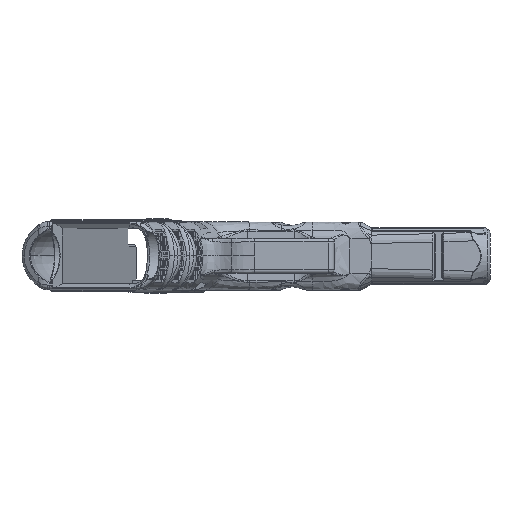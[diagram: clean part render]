
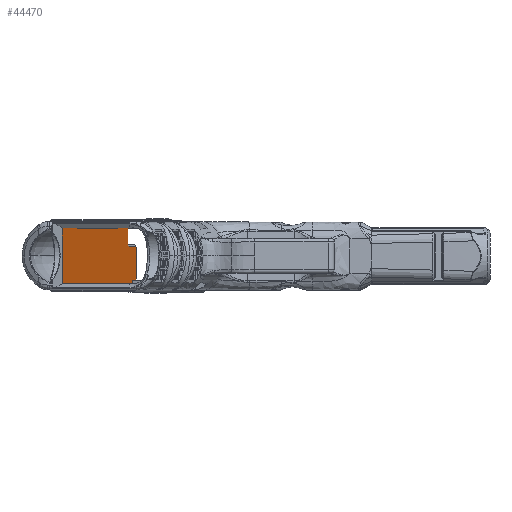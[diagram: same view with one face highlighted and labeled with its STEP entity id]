
A CAD part, top view. The second image highlights one B-rep face of the part: STEP entity #44470.
In plain terms, the highlighted planar face has unit normal (0.951, 0, 0.309).
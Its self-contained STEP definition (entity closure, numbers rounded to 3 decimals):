
#2195=LINE('',#99948,#4883);
#2961=LINE('',#152782,#5649);
#3145=LINE('',#160101,#5833);
#3148=LINE('',#160106,#5836);
#3153=LINE('',#160131,#5841);
#3154=LINE('',#160134,#5842);
#3155=LINE('',#160136,#5843);
#3156=LINE('',#160140,#5844);
#3157=LINE('',#160142,#5845);
#3158=LINE('',#160143,#5846);
#4883=VECTOR('',#52501,10.);
#5649=VECTOR('',#55797,10.);
#5833=VECTOR('',#56309,10.);
#5836=VECTOR('',#56316,10.);
#5841=VECTOR('',#56331,1000.);
#5842=VECTOR('',#56334,10.);
#5843=VECTOR('',#56335,10.);
#5844=VECTOR('',#56338,10.);
#5845=VECTOR('',#56339,10.);
#5846=VECTOR('',#56340,1000.);
#7071=PLANE('',#47829);
#8424=ELLIPSE('',#47830,0.536,0.51);
#10354=FACE_OUTER_BOUND('',#12789,.T.);
#12789=EDGE_LOOP('',(#39009,#39010,#39011,#39012,#39013,#39014,#39015,#39016,
#39017,#39018,#39019));
#18536=VERTEX_POINT('',#99830);
#18546=VERTEX_POINT('',#99929);
#19970=VERTEX_POINT('',#152779);
#19971=VERTEX_POINT('',#152781);
#20238=VERTEX_POINT('',#160095);
#20240=VERTEX_POINT('',#160099);
#20248=VERTEX_POINT('',#160133);
#20249=VERTEX_POINT('',#160135);
#20250=VERTEX_POINT('',#160137);
#20251=VERTEX_POINT('',#160139);
#20252=VERTEX_POINT('',#160141);
#24022=EDGE_CURVE('',#18536,#18546,#2195,.T.);
#26262=EDGE_CURVE('',#19970,#19971,#2961,.T.);
#26684=EDGE_CURVE('',#20238,#20240,#3145,.T.);
#26687=EDGE_CURVE('',#20240,#19971,#3148,.T.);
#26697=EDGE_CURVE('',#20238,#18536,#3153,.T.);
#26698=EDGE_CURVE('',#20248,#19970,#3154,.T.);
#26699=EDGE_CURVE('',#20249,#20248,#3155,.T.);
#26700=EDGE_CURVE('',#20250,#20249,#8424,.T.);
#26701=EDGE_CURVE('',#20251,#20250,#3156,.T.);
#26702=EDGE_CURVE('',#20252,#20251,#3157,.T.);
#26703=EDGE_CURVE('',#18546,#20252,#3158,.T.);
#39009=ORIENTED_EDGE('',*,*,#26697,.F.);
#39010=ORIENTED_EDGE('',*,*,#26684,.T.);
#39011=ORIENTED_EDGE('',*,*,#26687,.T.);
#39012=ORIENTED_EDGE('',*,*,#26262,.F.);
#39013=ORIENTED_EDGE('',*,*,#26698,.F.);
#39014=ORIENTED_EDGE('',*,*,#26699,.F.);
#39015=ORIENTED_EDGE('',*,*,#26700,.F.);
#39016=ORIENTED_EDGE('',*,*,#26701,.F.);
#39017=ORIENTED_EDGE('',*,*,#26702,.F.);
#39018=ORIENTED_EDGE('',*,*,#26703,.F.);
#39019=ORIENTED_EDGE('',*,*,#24022,.F.);
#44470=ADVANCED_FACE('',(#10354),#7071,.F.);
#47829=AXIS2_PLACEMENT_3D('',#160132,#56332,#56333);
#47830=AXIS2_PLACEMENT_3D('',#160138,#56336,#56337);
#52501=DIRECTION('',(0.,1.,0.));
#55797=DIRECTION('',(0.,-1.,0.));
#56309=DIRECTION('',(0.,1.,0.));
#56316=DIRECTION('',(0.309,0.,-0.951));
#56331=DIRECTION('',(-0.309,0.,0.951));
#56332=DIRECTION('center_axis',(-0.951,0.,
-0.309));
#56333=DIRECTION('ref_axis',(0.,1.,0.));
#56334=DIRECTION('',(-0.309,0.,0.951));
#56335=DIRECTION('',(0.,-1.,0.));
#56336=DIRECTION('center_axis',(-0.951,0.,
-0.309));
#56337=DIRECTION('ref_axis',(0.309,0.,-0.951));
#56338=DIRECTION('',(0.309,0.,-0.951));
#56339=DIRECTION('',(0.,-1.,0.));
#56340=DIRECTION('',(0.309,0.,-0.951));
#99830=CARTESIAN_POINT('',(2.236,-11.75,98.));
#99929=CARTESIAN_POINT('',(2.236,11.75,98.));
#99948=CARTESIAN_POINT('',(2.236,-18.375,98.));
#152779=CARTESIAN_POINT('',(33.331,-9.542,2.3));
#152781=CARTESIAN_POINT('',(33.331,-10.25,2.3));
#152782=CARTESIAN_POINT('',(33.331,-5.876,2.3));
#160095=CARTESIAN_POINT('',(31.8,-11.75,7.012));
#160099=CARTESIAN_POINT('',(31.8,-10.25,7.012));
#160101=CARTESIAN_POINT('',(31.8,-11.75,7.012));
#160106=CARTESIAN_POINT('',(33.225,-10.25,2.625));
#160131=CARTESIAN_POINT('',(33.829,-11.75,0.765));
#160132=CARTESIAN_POINT('Origin',(33.829,-11.75,0.765));
#160133=CARTESIAN_POINT('',(33.382,-9.542,2.141));
#160134=CARTESIAN_POINT('',(28.825,-9.542,16.167));
#160135=CARTESIAN_POINT('',(33.382,3.75,2.141));
#160136=CARTESIAN_POINT('',(33.382,-5.651,2.141));
#160137=CARTESIAN_POINT('',(33.216,4.26,2.651));
#160138=CARTESIAN_POINT('Origin',(33.216,3.75,2.651));
#160139=CARTESIAN_POINT('',(29.972,4.26,12.638));
#160140=CARTESIAN_POINT('',(34.619,4.26,-1.664));
#160141=CARTESIAN_POINT('',(29.972,11.75,12.638));
#160142=CARTESIAN_POINT('',(29.972,2.982,12.638));
#160143=CARTESIAN_POINT('',(30.125,11.75,12.165));
